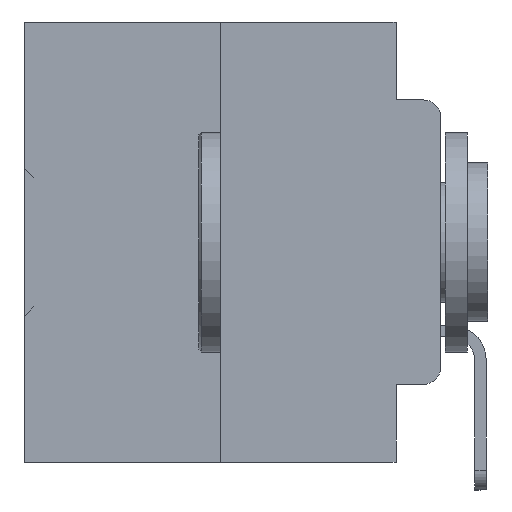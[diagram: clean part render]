
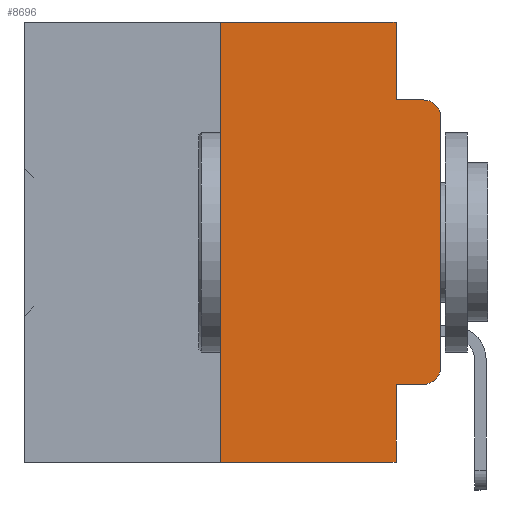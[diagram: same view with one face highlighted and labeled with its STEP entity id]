
A CAD part, left-side view. The second image highlights one B-rep face of the part: STEP entity #8696.
In plain terms, the highlighted planar face has unit normal (-1, 0, 0).
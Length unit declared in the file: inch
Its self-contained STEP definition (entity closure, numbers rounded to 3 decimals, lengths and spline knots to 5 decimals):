
#585 = ORIENTED_EDGE ( 'NONE', *, *, #38077, .T. ) ;
#2175 = DIRECTION ( 'NONE',  ( 0., -1., 0. ) ) ;
#3054 = ORIENTED_EDGE ( 'NONE', *, *, #35837, .F. ) ;
#3275 = DIRECTION ( 'NONE',  ( 0., 0., -1. ) ) ;
#3473 = DIRECTION ( 'NONE',  ( 0., -1., 0. ) ) ;
#4988 = LINE ( 'NONE', #14266, #12634 ) ;
#5118 = CARTESIAN_POINT ( 'NONE',  ( 0., 0.051, -0.0885 ) ) ;
#5573 = EDGE_LOOP ( 'NONE', ( #27882, #11984, #23291, #17255, #6598, #3054, #11113, #18973, #585, #38134 ) ) ;
#5710 = CARTESIAN_POINT ( 'NONE',  ( 0., 0.02, -0.1085 ) ) ;
#5727 = VERTEX_POINT ( 'NONE', #16939 ) ;
#6013 = AXIS2_PLACEMENT_3D ( 'NONE', #27367, #12621, #33864 ) ;
#6257 = CARTESIAN_POINT ( 'NONE',  ( 0., 0.02, -0.0885 ) ) ;
#6486 = CARTESIAN_POINT ( 'NONE',  ( 0., 0.051, 0. ) ) ;
#6598 = ORIENTED_EDGE ( 'NONE', *, *, #38259, .F. ) ;
#6875 = CARTESIAN_POINT ( 'NONE',  ( 0., 0.051, -0.0885 ) ) ;
#7413 = VECTOR ( 'NONE', #24947, 39.37008 ) ;
#7747 = CARTESIAN_POINT ( 'NONE',  ( 0., 0., -0.3915 ) ) ;
#8031 = AXIS2_PLACEMENT_3D ( 'NONE', #21190, #39076, #17872 ) ;
#8696 = ADVANCED_FACE ( 'NONE', ( #15488 ), #12486, .F. ) ;
#9555 = VERTEX_POINT ( 'NONE', #25581 ) ;
#9730 = DIRECTION ( 'NONE',  ( 0., -1., 0. ) ) ;
#10691 = VERTEX_POINT ( 'NONE', #6875 ) ;
#11113 = ORIENTED_EDGE ( 'NONE', *, *, #33337, .T. ) ;
#11612 = EDGE_CURVE ( 'NONE', #16554, #10691, #31444, .T. ) ;
#11623 = VERTEX_POINT ( 'NONE', #15465 ) ;
#11768 = CARTESIAN_POINT ( 'NONE',  ( 0., 0.051, -0.5 ) ) ;
#11827 = DIRECTION ( 'NONE',  ( -1., 0., 0. ) ) ;
#11984 = ORIENTED_EDGE ( 'NONE', *, *, #35455, .T. ) ;
#12486 = PLANE ( 'NONE',  #6013 ) ;
#12589 = VERTEX_POINT ( 'NONE', #11768 ) ;
#12621 = DIRECTION ( 'NONE',  ( 1., 0., 0. ) ) ;
#12634 = VECTOR ( 'NONE', #39032, 39.37008 ) ;
#12980 = CIRCLE ( 'NONE', #8031, 0.02 ) ;
#13068 = CARTESIAN_POINT ( 'NONE',  ( 0., 0.051, 0. ) ) ;
#13884 = VECTOR ( 'NONE', #9730, 39.37008 ) ;
#14266 = CARTESIAN_POINT ( 'NONE',  ( 0., 0.473, -0.5 ) ) ;
#15086 = LINE ( 'NONE', #6486, #37836 ) ;
#15465 = CARTESIAN_POINT ( 'NONE',  ( 0., 0.051, -0.4115 ) ) ;
#15488 = FACE_OUTER_BOUND ( 'NONE', #5573, .T. ) ;
#16554 = VERTEX_POINT ( 'NONE', #13068 ) ;
#16939 = CARTESIAN_POINT ( 'NONE',  ( 0., 0.25, -0.5 ) ) ;
#16987 = CIRCLE ( 'NONE', #22293, 0.02 ) ;
#17255 = ORIENTED_EDGE ( 'NONE', *, *, #11612, .F. ) ;
#17680 = EDGE_CURVE ( 'NONE', #24782, #30092, #37960, .T. ) ;
#17872 = DIRECTION ( 'NONE',  ( 0., 0., -1. ) ) ;
#18175 = DIRECTION ( 'NONE',  ( 0., 0., 1. ) ) ;
#18470 = EDGE_CURVE ( 'NONE', #11623, #12589, #15086, .T. ) ;
#18973 = ORIENTED_EDGE ( 'NONE', *, *, #18470, .F. ) ;
#19124 = CARTESIAN_POINT ( 'NONE',  ( 0., 0.25, 0. ) ) ;
#21190 = CARTESIAN_POINT ( 'NONE',  ( 0., 0.02, -0.3915 ) ) ;
#21418 = DIRECTION ( 'NONE',  ( 0., 0., -1. ) ) ;
#22293 = AXIS2_PLACEMENT_3D ( 'NONE', #5710, #11827, #33077 ) ;
#23291 = ORIENTED_EDGE ( 'NONE', *, *, #36140, .F. ) ;
#23842 = LINE ( 'NONE', #36989, #30952 ) ;
#24782 = VERTEX_POINT ( 'NONE', #7747 ) ;
#24900 = CARTESIAN_POINT ( 'NONE',  ( 0., 0.473, 0. ) ) ;
#24947 = DIRECTION ( 'NONE',  ( 0., 0., 1. ) ) ;
#25186 = VERTEX_POINT ( 'NONE', #28216 ) ;
#25581 = CARTESIAN_POINT ( 'NONE',  ( 0., 0.02, -0.4115 ) ) ;
#27367 = CARTESIAN_POINT ( 'NONE',  ( 0., 0.473, 0. ) ) ;
#27882 = ORIENTED_EDGE ( 'NONE', *, *, #17680, .T. ) ;
#28216 = CARTESIAN_POINT ( 'NONE',  ( 0., 0.25, 0. ) ) ;
#29237 = EDGE_CURVE ( 'NONE', #9555, #24782, #12980, .T. ) ;
#29286 = VECTOR ( 'NONE', #2175, 39.37008 ) ;
#29774 = LINE ( 'NONE', #19124, #7413 ) ;
#30092 = VERTEX_POINT ( 'NONE', #37718 ) ;
#30525 = CARTESIAN_POINT ( 'NONE',  ( 0., 0., 0. ) ) ;
#30952 = VECTOR ( 'NONE', #3473, 39.37008 ) ;
#31444 = LINE ( 'NONE', #33745, #39009 ) ;
#31931 = LINE ( 'NONE', #24900, #13884 ) ;
#31934 = VERTEX_POINT ( 'NONE', #6257 ) ;
#32585 = LINE ( 'NONE', #5118, #29286 ) ;
#33077 = DIRECTION ( 'NONE',  ( 0., 0., -1. ) ) ;
#33337 = EDGE_CURVE ( 'NONE', #5727, #12589, #4988, .T. ) ;
#33745 = CARTESIAN_POINT ( 'NONE',  ( 0., 0.051, 0. ) ) ;
#33864 = DIRECTION ( 'NONE',  ( 0., 0., -1. ) ) ;
#35455 = EDGE_CURVE ( 'NONE', #30092, #31934, #16987, .T. ) ;
#35837 = EDGE_CURVE ( 'NONE', #5727, #25186, #29774, .T. ) ;
#36140 = EDGE_CURVE ( 'NONE', #10691, #31934, #32585, .T. ) ;
#36989 = CARTESIAN_POINT ( 'NONE',  ( 0., 0.051, -0.4115 ) ) ;
#37459 = VECTOR ( 'NONE', #18175, 39.37008 ) ;
#37718 = CARTESIAN_POINT ( 'NONE',  ( 0., 0., -0.1085 ) ) ;
#37836 = VECTOR ( 'NONE', #3275, 39.37008 ) ;
#37960 = LINE ( 'NONE', #30525, #37459 ) ;
#38077 = EDGE_CURVE ( 'NONE', #11623, #9555, #23842, .T. ) ;
#38134 = ORIENTED_EDGE ( 'NONE', *, *, #29237, .T. ) ;
#38259 = EDGE_CURVE ( 'NONE', #25186, #16554, #31931, .T. ) ;
#39009 = VECTOR ( 'NONE', #21418, 39.37008 ) ;
#39032 = DIRECTION ( 'NONE',  ( 0., -1., 0. ) ) ;
#39076 = DIRECTION ( 'NONE',  ( -1., 0., 0. ) ) ;
